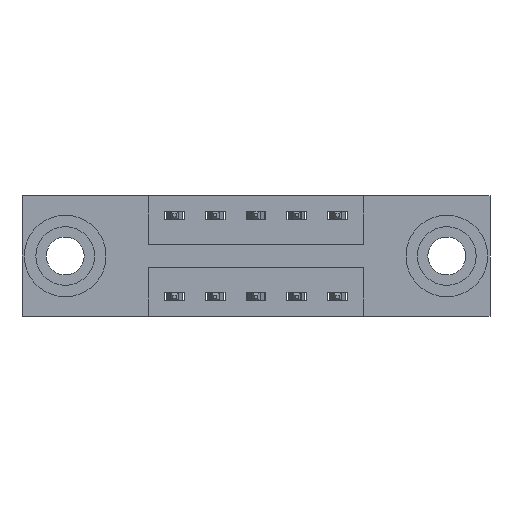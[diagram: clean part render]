
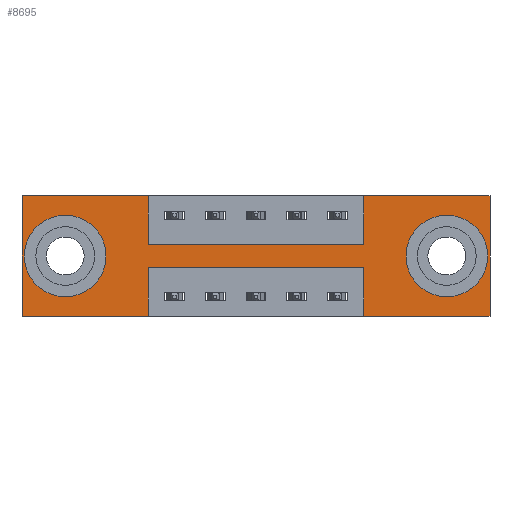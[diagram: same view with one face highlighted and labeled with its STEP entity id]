
A CAD part, front view. The second image highlights one B-rep face of the part: STEP entity #8695.
In plain terms, the highlighted planar face has unit normal (0, -1, 0).
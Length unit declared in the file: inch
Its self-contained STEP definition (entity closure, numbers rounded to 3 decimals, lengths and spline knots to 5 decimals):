
#34 = FACE_BOUND ( 'NONE', #6201, .T. ) ;
#64 = VERTEX_POINT ( 'NONE', #7674 ) ;
#129 = EDGE_CURVE ( 'NONE', #4728, #6372, #2633, .T. ) ;
#190 = EDGE_CURVE ( 'NONE', #4653, #5524, #5620, .T. ) ;
#193 = ORIENTED_EDGE ( 'NONE', *, *, #538, .T. ) ;
#538 = EDGE_CURVE ( 'NONE', #1247, #3217, #8035, .T. ) ;
#659 = VERTEX_POINT ( 'NONE', #7509 ) ;
#736 = CARTESIAN_POINT ( 'NONE',  ( 0.3875, 0., -0.37 ) ) ;
#740 = AXIS2_PLACEMENT_3D ( 'NONE', #5013, #2857, #7845 ) ;
#950 = VERTEX_POINT ( 'NONE', #6769 ) ;
#1005 = CARTESIAN_POINT ( 'NONE',  ( 0.1325, 0., -0.185 ) ) ;
#1073 = CARTESIAN_POINT ( 'NONE',  ( 0., 0., 0. ) ) ;
#1078 = CARTESIAN_POINT ( 'NONE',  ( 0., 0., 0. ) ) ;
#1170 = DIRECTION ( 'NONE',  ( 1., 0., 0. ) ) ;
#1198 = DIRECTION ( 'NONE',  ( 0., 0., -1. ) ) ;
#1238 = VERTEX_POINT ( 'NONE', #8400 ) ;
#1247 = VERTEX_POINT ( 'NONE', #8390 ) ;
#1340 = ORIENTED_EDGE ( 'NONE', *, *, #7305, .F. ) ;
#1345 = DIRECTION ( 'NONE',  ( 1., 0., 0. ) ) ;
#1431 = EDGE_CURVE ( 'NONE', #5524, #4703, #4437, .T. ) ;
#1504 = CARTESIAN_POINT ( 'NONE',  ( 0., 0., 0. ) ) ;
#1616 = CARTESIAN_POINT ( 'NONE',  ( 1.3025, 0., -0.185 ) ) ;
#1648 = VECTOR ( 'NONE', #5520, 39.37008 ) ;
#1702 = ORIENTED_EDGE ( 'NONE', *, *, #5594, .F. ) ;
#1729 = CARTESIAN_POINT ( 'NONE',  ( 0.3875, 0., -0.37 ) ) ;
#1732 = DIRECTION ( 'NONE',  ( 0., -1., 0. ) ) ;
#1757 = CARTESIAN_POINT ( 'NONE',  ( 0.3875, 0., 0. ) ) ;
#1805 = LINE ( 'NONE', #1757, #7108 ) ;
#1894 = LINE ( 'NONE', #7651, #1648 ) ;
#1906 = CARTESIAN_POINT ( 'NONE',  ( 1.435, 0., 0. ) ) ;
#2002 = CARTESIAN_POINT ( 'NONE',  ( 1.0475, 0., -0.15 ) ) ;
#2069 = CARTESIAN_POINT ( 'NONE',  ( 0., 0., -0.37 ) ) ;
#2256 = FACE_BOUND ( 'NONE', #4881, .T. ) ;
#2355 = EDGE_CURVE ( 'NONE', #4703, #4878, #5776, .T. ) ;
#2403 = PLANE ( 'NONE',  #3989 ) ;
#2420 = ORIENTED_EDGE ( 'NONE', *, *, #8572, .F. ) ;
#2423 = ORIENTED_EDGE ( 'NONE', *, *, #1431, .F. ) ;
#2470 = CARTESIAN_POINT ( 'NONE',  ( 1.3025, 0., -0.185 ) ) ;
#2596 = ORIENTED_EDGE ( 'NONE', *, *, #8596, .F. ) ;
#2608 = AXIS2_PLACEMENT_3D ( 'NONE', #1616, #8882, #6684 ) ;
#2626 = VERTEX_POINT ( 'NONE', #7457 ) ;
#2633 = LINE ( 'NONE', #3481, #7600 ) ;
#2735 = EDGE_CURVE ( 'NONE', #3217, #1247, #7860, .T. ) ;
#2847 = VECTOR ( 'NONE', #3572, 39.37008 ) ;
#2857 = DIRECTION ( 'NONE',  ( 0., 1., 0. ) ) ;
#2948 = CIRCLE ( 'NONE', #2608, 0.078 ) ;
#2964 = ORIENTED_EDGE ( 'NONE', *, *, #8060, .F. ) ;
#3113 = CARTESIAN_POINT ( 'NONE',  ( 1.0475, 0., 0. ) ) ;
#3217 = VERTEX_POINT ( 'NONE', #3375 ) ;
#3230 = DIRECTION ( 'NONE',  ( 0., 0., -1. ) ) ;
#3375 = CARTESIAN_POINT ( 'NONE',  ( 0.1325, 0., -0.263 ) ) ;
#3481 = CARTESIAN_POINT ( 'NONE',  ( 0.3875, 0., -0.22 ) ) ;
#3489 = CARTESIAN_POINT ( 'NONE',  ( 1.0475, 0., 0. ) ) ;
#3515 = DIRECTION ( 'NONE',  ( 0., 0., 1. ) ) ;
#3560 = LINE ( 'NONE', #1729, #8706 ) ;
#3572 = DIRECTION ( 'NONE',  ( -1., 0., 0. ) ) ;
#3595 = VECTOR ( 'NONE', #1170, 39.37008 ) ;
#3598 = AXIS2_PLACEMENT_3D ( 'NONE', #2470, #5667, #8836 ) ;
#3603 = VERTEX_POINT ( 'NONE', #1504 ) ;
#3613 = DIRECTION ( 'NONE',  ( 0., 0., -1. ) ) ;
#3673 = CARTESIAN_POINT ( 'NONE',  ( 1.3025, 0., -0.107 ) ) ;
#3733 = EDGE_CURVE ( 'NONE', #5912, #1238, #2948, .T. ) ;
#3827 = ORIENTED_EDGE ( 'NONE', *, *, #4030, .F. ) ;
#3944 = CARTESIAN_POINT ( 'NONE',  ( 0.3875, 0., -0.22 ) ) ;
#3989 = AXIS2_PLACEMENT_3D ( 'NONE', #5373, #1732, #1198 ) ;
#4030 = EDGE_CURVE ( 'NONE', #3603, #64, #4194, .T. ) ;
#4051 = AXIS2_PLACEMENT_3D ( 'NONE', #1005, #6376, #6576 ) ;
#4194 = LINE ( 'NONE', #1078, #4795 ) ;
#4352 = LINE ( 'NONE', #8769, #6417 ) ;
#4384 = ORIENTED_EDGE ( 'NONE', *, *, #3733, .T. ) ;
#4437 = LINE ( 'NONE', #1073, #3595 ) ;
#4455 = VECTOR ( 'NONE', #5475, 39.37008 ) ;
#4653 = VERTEX_POINT ( 'NONE', #2002 ) ;
#4703 = VERTEX_POINT ( 'NONE', #7703 ) ;
#4721 = ORIENTED_EDGE ( 'NONE', *, *, #190, .F. ) ;
#4728 = VERTEX_POINT ( 'NONE', #6013 ) ;
#4795 = VECTOR ( 'NONE', #1345, 39.37008 ) ;
#4825 = VECTOR ( 'NONE', #8251, 39.37008 ) ;
#4848 = ORIENTED_EDGE ( 'NONE', *, *, #2735, .T. ) ;
#4878 = VERTEX_POINT ( 'NONE', #6894 ) ;
#4881 = EDGE_LOOP ( 'NONE', ( #4384, #6438 ) ) ;
#5013 = CARTESIAN_POINT ( 'NONE',  ( 0.1325, 0., -0.185 ) ) ;
#5027 = ORIENTED_EDGE ( 'NONE', *, *, #129, .F. ) ;
#5042 = LINE ( 'NONE', #8178, #4825 ) ;
#5056 = ORIENTED_EDGE ( 'NONE', *, *, #6977, .F. ) ;
#5224 = DIRECTION ( 'NONE',  ( 0., 0., -1. ) ) ;
#5373 = CARTESIAN_POINT ( 'NONE',  ( 0., 0., -0.37 ) ) ;
#5475 = DIRECTION ( 'NONE',  ( 0., 0., 1. ) ) ;
#5520 = DIRECTION ( 'NONE',  ( 0., 0., 1. ) ) ;
#5524 = VERTEX_POINT ( 'NONE', #3489 ) ;
#5537 = FACE_OUTER_BOUND ( 'NONE', #5852, .T. ) ;
#5581 = ORIENTED_EDGE ( 'NONE', *, *, #7393, .F. ) ;
#5594 = EDGE_CURVE ( 'NONE', #2626, #4653, #5042, .T. ) ;
#5620 = LINE ( 'NONE', #3113, #6321 ) ;
#5667 = DIRECTION ( 'NONE',  ( 0., 1., 0. ) ) ;
#5776 = LINE ( 'NONE', #1906, #7694 ) ;
#5852 = EDGE_LOOP ( 'NONE', ( #2596, #5027, #2420, #1340, #5917, #2423, #4721, #1702, #5581, #3827, #2964, #5056 ) ) ;
#5866 = DIRECTION ( 'NONE',  ( -1., 0., 0. ) ) ;
#5912 = VERTEX_POINT ( 'NONE', #3673 ) ;
#5917 = ORIENTED_EDGE ( 'NONE', *, *, #2355, .F. ) ;
#6013 = CARTESIAN_POINT ( 'NONE',  ( 1.0475, 0., -0.22 ) ) ;
#6176 = VERTEX_POINT ( 'NONE', #736 ) ;
#6201 = EDGE_LOOP ( 'NONE', ( #193, #4848 ) ) ;
#6321 = VECTOR ( 'NONE', #3515, 39.37008 ) ;
#6372 = VERTEX_POINT ( 'NONE', #3944 ) ;
#6376 = DIRECTION ( 'NONE',  ( 0., 1., 0. ) ) ;
#6417 = VECTOR ( 'NONE', #6440, 39.37008 ) ;
#6438 = ORIENTED_EDGE ( 'NONE', *, *, #6866, .T. ) ;
#6440 = DIRECTION ( 'NONE',  ( -1., 0., 0. ) ) ;
#6521 = LINE ( 'NONE', #2069, #2847 ) ;
#6576 = DIRECTION ( 'NONE',  ( 0., 0., 1. ) ) ;
#6684 = DIRECTION ( 'NONE',  ( 0., 0., -1. ) ) ;
#6769 = CARTESIAN_POINT ( 'NONE',  ( 0., 0., -0.37 ) ) ;
#6866 = EDGE_CURVE ( 'NONE', #1238, #5912, #8637, .T. ) ;
#6894 = CARTESIAN_POINT ( 'NONE',  ( 1.435, 0., -0.37 ) ) ;
#6977 = EDGE_CURVE ( 'NONE', #6176, #950, #6521, .T. ) ;
#7108 = VECTOR ( 'NONE', #3613, 39.37008 ) ;
#7305 = EDGE_CURVE ( 'NONE', #4878, #659, #4352, .T. ) ;
#7393 = EDGE_CURVE ( 'NONE', #64, #2626, #1805, .T. ) ;
#7457 = CARTESIAN_POINT ( 'NONE',  ( 0.3875, 0., -0.15 ) ) ;
#7509 = CARTESIAN_POINT ( 'NONE',  ( 1.0475, 0., -0.37 ) ) ;
#7600 = VECTOR ( 'NONE', #5866, 39.37008 ) ;
#7651 = CARTESIAN_POINT ( 'NONE',  ( 1.0475, 0., -0.37 ) ) ;
#7674 = CARTESIAN_POINT ( 'NONE',  ( 0.3875, 0., 0. ) ) ;
#7694 = VECTOR ( 'NONE', #5224, 39.37008 ) ;
#7703 = CARTESIAN_POINT ( 'NONE',  ( 1.435, 0., 0. ) ) ;
#7845 = DIRECTION ( 'NONE',  ( 0., 0., 1. ) ) ;
#7860 = CIRCLE ( 'NONE', #740, 0.078 ) ;
#8035 = CIRCLE ( 'NONE', #4051, 0.078 ) ;
#8060 = EDGE_CURVE ( 'NONE', #950, #3603, #8910, .T. ) ;
#8178 = CARTESIAN_POINT ( 'NONE',  ( 0.3875, 0., -0.15 ) ) ;
#8251 = DIRECTION ( 'NONE',  ( 1., 0., 0. ) ) ;
#8273 = CARTESIAN_POINT ( 'NONE',  ( 0., 0., 0. ) ) ;
#8390 = CARTESIAN_POINT ( 'NONE',  ( 0.1325, 0., -0.107 ) ) ;
#8400 = CARTESIAN_POINT ( 'NONE',  ( 1.3025, 0., -0.263 ) ) ;
#8572 = EDGE_CURVE ( 'NONE', #659, #4728, #1894, .T. ) ;
#8596 = EDGE_CURVE ( 'NONE', #6372, #6176, #3560, .T. ) ;
#8637 = CIRCLE ( 'NONE', #3598, 0.078 ) ;
#8695 = ADVANCED_FACE ( 'NONE', ( #2256, #34, #5537 ), #2403, .T. ) ;
#8706 = VECTOR ( 'NONE', #3230, 39.37008 ) ;
#8769 = CARTESIAN_POINT ( 'NONE',  ( 0., 0., -0.37 ) ) ;
#8836 = DIRECTION ( 'NONE',  ( 0., 0., -1. ) ) ;
#8882 = DIRECTION ( 'NONE',  ( 0., 1., 0. ) ) ;
#8910 = LINE ( 'NONE', #8273, #4455 ) ;
